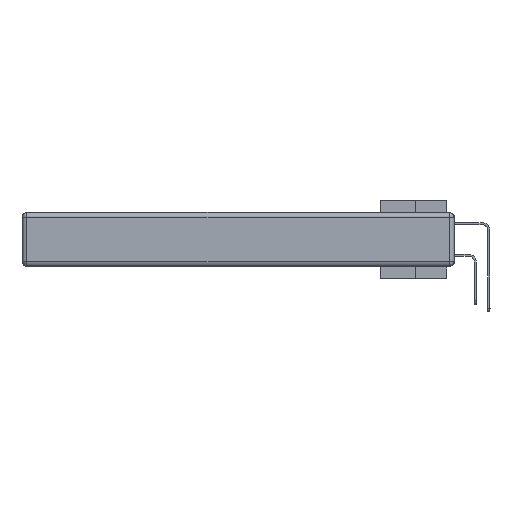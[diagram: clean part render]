
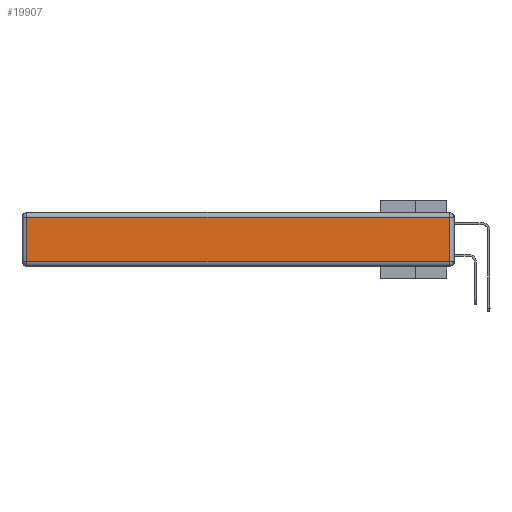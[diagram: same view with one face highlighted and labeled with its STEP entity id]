
A CAD part, left-side view. The second image highlights one B-rep face of the part: STEP entity #19907.
In plain terms, the highlighted planar face has unit normal (-1, 0, 0).
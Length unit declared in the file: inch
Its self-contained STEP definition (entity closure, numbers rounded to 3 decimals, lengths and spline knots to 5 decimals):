
#4762 = LINE ( 'NONE', #33907, #27398 ) ;
#5337 = EDGE_CURVE ( 'NONE', #39059, #18227, #22692, .T. ) ;
#5797 = CARTESIAN_POINT ( 'NONE',  ( 0., 0.03, -0.313 ) ) ;
#7581 = LINE ( 'NONE', #13769, #38210 ) ;
#9900 = VERTEX_POINT ( 'NONE', #5797 ) ;
#10906 = EDGE_LOOP ( 'NONE', ( #34209, #39691, #28399, #39733 ) ) ;
#12742 = DIRECTION ( 'NONE',  ( -1., 0., 0. ) ) ;
#13143 = EDGE_CURVE ( 'NONE', #18227, #9900, #4762, .T. ) ;
#13163 = DIRECTION ( 'NONE',  ( 0., 0., 1. ) ) ;
#13498 = DIRECTION ( 'NONE',  ( 0., 0., -1. ) ) ;
#13769 = CARTESIAN_POINT ( 'NONE',  ( 0., 0.03, -0.343 ) ) ;
#17648 = VERTEX_POINT ( 'NONE', #28883 ) ;
#18227 = VERTEX_POINT ( 'NONE', #20451 ) ;
#18911 = CARTESIAN_POINT ( 'NONE',  ( 0., 0., -0.343 ) ) ;
#19907 = ADVANCED_FACE ( 'NONE', ( #29006 ), #42106, .T. ) ;
#20451 = CARTESIAN_POINT ( 'NONE',  ( 0., 2.72, -0.313 ) ) ;
#22692 = LINE ( 'NONE', #33204, #27677 ) ;
#26615 = DIRECTION ( 'NONE',  ( 0., 0., 1. ) ) ;
#27397 = EDGE_CURVE ( 'NONE', #17648, #39059, #34208, .T. ) ;
#27398 = VECTOR ( 'NONE', #34729, 39.37008 ) ;
#27677 = VECTOR ( 'NONE', #13498, 39.37008 ) ;
#28399 = ORIENTED_EDGE ( 'NONE', *, *, #27397, .T. ) ;
#28883 = CARTESIAN_POINT ( 'NONE',  ( 0., 0.03, -0.03 ) ) ;
#29006 = FACE_OUTER_BOUND ( 'NONE', #10906, .T. ) ;
#31681 = EDGE_CURVE ( 'NONE', #9900, #17648, #7581, .T. ) ;
#33204 = CARTESIAN_POINT ( 'NONE',  ( 0., 2.72, -0.343 ) ) ;
#33578 = DIRECTION ( 'NONE',  ( 0., 1., 0. ) ) ;
#33907 = CARTESIAN_POINT ( 'NONE',  ( 0., 0., -0.313 ) ) ;
#34208 = LINE ( 'NONE', #37637, #40984 ) ;
#34209 = ORIENTED_EDGE ( 'NONE', *, *, #13143, .T. ) ;
#34729 = DIRECTION ( 'NONE',  ( 0., -1., 0. ) ) ;
#37637 = CARTESIAN_POINT ( 'NONE',  ( 0., 2.75, -0.03 ) ) ;
#38210 = VECTOR ( 'NONE', #26615, 39.37008 ) ;
#39059 = VERTEX_POINT ( 'NONE', #41489 ) ;
#39691 = ORIENTED_EDGE ( 'NONE', *, *, #31681, .T. ) ;
#39733 = ORIENTED_EDGE ( 'NONE', *, *, #5337, .T. ) ;
#40692 = AXIS2_PLACEMENT_3D ( 'NONE', #18911, #12742, #13163 ) ;
#40984 = VECTOR ( 'NONE', #33578, 39.37008 ) ;
#41489 = CARTESIAN_POINT ( 'NONE',  ( 0., 2.72, -0.03 ) ) ;
#42106 = PLANE ( 'NONE',  #40692 ) ;
